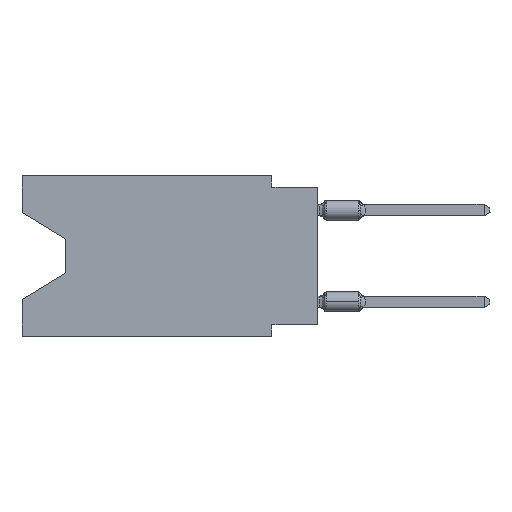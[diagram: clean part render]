
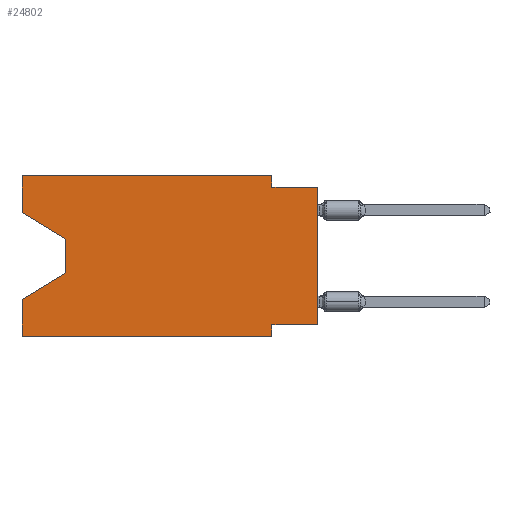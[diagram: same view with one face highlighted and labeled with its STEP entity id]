
A CAD part, left-side view. The second image highlights one B-rep face of the part: STEP entity #24802.
In plain terms, the highlighted planar face has unit normal (-1, 0, 0).
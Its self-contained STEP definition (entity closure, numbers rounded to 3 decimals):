
#71 = EDGE_CURVE ( 'NONE', #38669, #20505, #30761, .T. ) ;
#401 = FACE_OUTER_BOUND ( 'NONE', #18172, .T. ) ;
#1538 = ORIENTED_EDGE ( 'NONE', *, *, #71, .F. ) ;
#2650 = VECTOR ( 'NONE', #27547, 1000. ) ;
#4312 = DIRECTION ( 'NONE',  ( 0., 0., 1. ) ) ;
#4346 = CARTESIAN_POINT ( 'NONE',  ( 0., 16.383, 0. ) ) ;
#4560 = DIRECTION ( 'NONE',  ( 0., -0.855, -0.519 ) ) ;
#4810 = LINE ( 'NONE', #29814, #14419 ) ;
#5515 = EDGE_CURVE ( 'NONE', #22201, #34243, #4810, .T. ) ;
#5730 = ORIENTED_EDGE ( 'NONE', *, *, #19334, .F. ) ;
#5742 = CARTESIAN_POINT ( 'NONE',  ( 0., 2.54, -0.635 ) ) ;
#5982 = CARTESIAN_POINT ( 'NONE',  ( 0., 16.383, -2.038 ) ) ;
#6202 = VECTOR ( 'NONE', #25476, 1000. ) ;
#6484 = DIRECTION ( 'NONE',  ( 0., 0.855, -0.519 ) ) ;
#7107 = VECTOR ( 'NONE', #40974, 1000. ) ;
#7690 = AXIS2_PLACEMENT_3D ( 'NONE', #48106, #13045, #21956 ) ;
#8424 = ORIENTED_EDGE ( 'NONE', *, *, #5515, .F. ) ;
#8486 = VERTEX_POINT ( 'NONE', #5982 ) ;
#8614 = CARTESIAN_POINT ( 'NONE',  ( 0., 0., 0. ) ) ;
#10022 = CARTESIAN_POINT ( 'NONE',  ( 0., 16.383, -8.89 ) ) ;
#11777 = CARTESIAN_POINT ( 'NONE',  ( 0., 0., -8.255 ) ) ;
#11784 = LINE ( 'NONE', #24159, #12502 ) ;
#12502 = VECTOR ( 'NONE', #55484, 1000. ) ;
#13045 = DIRECTION ( 'NONE',  ( 1., 0., 0. ) ) ;
#13205 = LINE ( 'NONE', #8614, #17105 ) ;
#14419 = VECTOR ( 'NONE', #47357, 1000. ) ;
#15606 = EDGE_CURVE ( 'NONE', #34243, #20153, #11784, .T. ) ;
#16554 = CARTESIAN_POINT ( 'NONE',  ( 0., 16.383, 0. ) ) ;
#16573 = ORIENTED_EDGE ( 'NONE', *, *, #30801, .T. ) ;
#17105 = VECTOR ( 'NONE', #4312, 1000. ) ;
#17175 = VECTOR ( 'NONE', #4560, 1000. ) ;
#17325 = ORIENTED_EDGE ( 'NONE', *, *, #15606, .F. ) ;
#17364 = EDGE_CURVE ( 'NONE', #40373, #36536, #50794, .T. ) ;
#17686 = EDGE_CURVE ( 'NONE', #37021, #20505, #49873, .T. ) ;
#18172 = EDGE_LOOP ( 'NONE', ( #33412, #16573, #44403, #1538, #18791, #51692, #20470, #20510, #17325, #8424, #5730, #42265 ) ) ;
#18249 = CARTESIAN_POINT ( 'NONE',  ( 0., 2.54, -8.255 ) ) ;
#18791 = ORIENTED_EDGE ( 'NONE', *, *, #50327, .T. ) ;
#19334 = EDGE_CURVE ( 'NONE', #42333, #22201, #32284, .T. ) ;
#19487 = CARTESIAN_POINT ( 'NONE',  ( 0., 0., -0.635 ) ) ;
#20130 = LINE ( 'NONE', #11777, #43853 ) ;
#20153 = VERTEX_POINT ( 'NONE', #19487 ) ;
#20470 = ORIENTED_EDGE ( 'NONE', *, *, #31694, .F. ) ;
#20505 = VERTEX_POINT ( 'NONE', #44733 ) ;
#20510 = ORIENTED_EDGE ( 'NONE', *, *, #45563, .T. ) ;
#21860 = DIRECTION ( 'NONE',  ( 0., 0., 1. ) ) ;
#21956 = DIRECTION ( 'NONE',  ( 0., 0., -1. ) ) ;
#22201 = VERTEX_POINT ( 'NONE', #51229 ) ;
#22936 = CARTESIAN_POINT ( 'NONE',  ( 0., 16.383, -2.038 ) ) ;
#23223 = LINE ( 'NONE', #10022, #2650 ) ;
#23665 = DIRECTION ( 'NONE',  ( 0., -1., 0. ) ) ;
#24159 = CARTESIAN_POINT ( 'NONE',  ( 0., 0., -0.635 ) ) ;
#24802 = ADVANCED_FACE ( 'NONE', ( #401 ), #48409, .F. ) ;
#25183 = LINE ( 'NONE', #16554, #6202 ) ;
#25476 = DIRECTION ( 'NONE',  ( 0., 0., 1. ) ) ;
#27202 = CARTESIAN_POINT ( 'NONE',  ( 0., 16.383, 0. ) ) ;
#27547 = DIRECTION ( 'NONE',  ( 0., -1., 0. ) ) ;
#28153 = VERTEX_POINT ( 'NONE', #42861 ) ;
#28291 = CARTESIAN_POINT ( 'NONE',  ( 0., 16.383, -8.89 ) ) ;
#28969 = EDGE_CURVE ( 'NONE', #8486, #42103, #49079, .T. ) ;
#29814 = CARTESIAN_POINT ( 'NONE',  ( 0., 2.54, 0. ) ) ;
#30761 = LINE ( 'NONE', #4346, #30980 ) ;
#30801 = EDGE_CURVE ( 'NONE', #42103, #37021, #54489, .T. ) ;
#30980 = VECTOR ( 'NONE', #21860, 1000. ) ;
#31694 = EDGE_CURVE ( 'NONE', #28153, #40373, #20130, .T. ) ;
#32284 = LINE ( 'NONE', #49246, #36437 ) ;
#33412 = ORIENTED_EDGE ( 'NONE', *, *, #28969, .T. ) ;
#33462 = CARTESIAN_POINT ( 'NONE',  ( 0., 13.97, -3.505 ) ) ;
#34111 = CARTESIAN_POINT ( 'NONE',  ( 0., 13.97, -3.505 ) ) ;
#34243 = VERTEX_POINT ( 'NONE', #5742 ) ;
#34949 = DIRECTION ( 'NONE',  ( 0., 1., 0. ) ) ;
#36198 = EDGE_CURVE ( 'NONE', #8486, #42333, #25183, .T. ) ;
#36437 = VECTOR ( 'NONE', #23665, 1000. ) ;
#36536 = VERTEX_POINT ( 'NONE', #37220 ) ;
#37021 = VERTEX_POINT ( 'NONE', #54811 ) ;
#37220 = CARTESIAN_POINT ( 'NONE',  ( 0., 2.54, -8.89 ) ) ;
#38669 = VERTEX_POINT ( 'NONE', #28291 ) ;
#40373 = VERTEX_POINT ( 'NONE', #18249 ) ;
#40974 = DIRECTION ( 'NONE',  ( 0., 0., -1. ) ) ;
#42103 = VERTEX_POINT ( 'NONE', #34111 ) ;
#42265 = ORIENTED_EDGE ( 'NONE', *, *, #36198, .F. ) ;
#42333 = VERTEX_POINT ( 'NONE', #27202 ) ;
#42359 = VECTOR ( 'NONE', #6484, 1000. ) ;
#42861 = CARTESIAN_POINT ( 'NONE',  ( 0., 0., -8.255 ) ) ;
#43853 = VECTOR ( 'NONE', #34949, 1000. ) ;
#44403 = ORIENTED_EDGE ( 'NONE', *, *, #17686, .T. ) ;
#44733 = CARTESIAN_POINT ( 'NONE',  ( 0., 16.383, -6.852 ) ) ;
#45073 = CARTESIAN_POINT ( 'NONE',  ( 0., 2.54, -8.89 ) ) ;
#45563 = EDGE_CURVE ( 'NONE', #28153, #20153, #13205, .T. ) ;
#47357 = DIRECTION ( 'NONE',  ( 0., 0., -1. ) ) ;
#48106 = CARTESIAN_POINT ( 'NONE',  ( 0., 16.383, 0. ) ) ;
#48409 = PLANE ( 'NONE',  #7690 ) ;
#48762 = VECTOR ( 'NONE', #49664, 1000. ) ;
#49079 = LINE ( 'NONE', #22936, #17175 ) ;
#49246 = CARTESIAN_POINT ( 'NONE',  ( 0., 16.383, 0. ) ) ;
#49664 = DIRECTION ( 'NONE',  ( 0., 0., -1. ) ) ;
#49873 = LINE ( 'NONE', #54481, #42359 ) ;
#50327 = EDGE_CURVE ( 'NONE', #38669, #36536, #23223, .T. ) ;
#50794 = LINE ( 'NONE', #45073, #48762 ) ;
#51229 = CARTESIAN_POINT ( 'NONE',  ( 0., 2.54, 0. ) ) ;
#51692 = ORIENTED_EDGE ( 'NONE', *, *, #17364, .F. ) ;
#54481 = CARTESIAN_POINT ( 'NONE',  ( 0., 13.97, -5.385 ) ) ;
#54489 = LINE ( 'NONE', #33462, #7107 ) ;
#54811 = CARTESIAN_POINT ( 'NONE',  ( 0., 13.97, -5.385 ) ) ;
#55484 = DIRECTION ( 'NONE',  ( 0., -1., 0. ) ) ;
